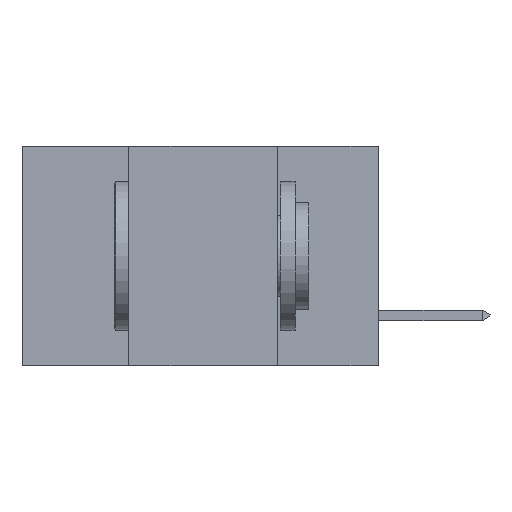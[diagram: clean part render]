
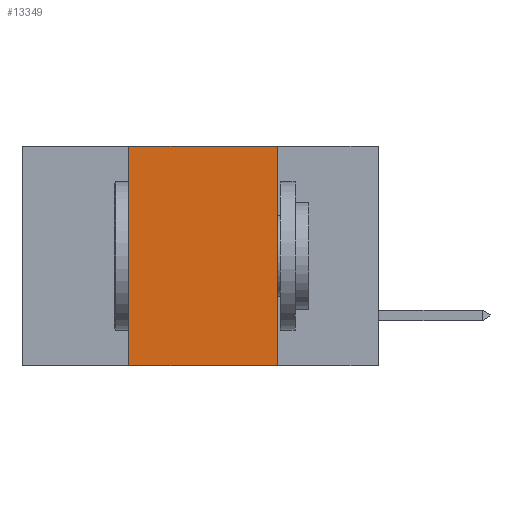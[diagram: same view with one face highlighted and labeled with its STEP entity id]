
A CAD part, left-side view. The second image highlights one B-rep face of the part: STEP entity #13349.
In plain terms, the highlighted planar face has unit normal (-1, 0, 0).
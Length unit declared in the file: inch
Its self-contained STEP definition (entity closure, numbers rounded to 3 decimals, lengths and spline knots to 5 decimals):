
#490 = DIRECTION ( 'NONE',  ( 0., 0., -1. ) ) ;
#607 = ORIENTED_EDGE ( 'NONE', *, *, #9971, .F. ) ;
#1518 = VECTOR ( 'NONE', #14403, 39.37008 ) ;
#1872 = CARTESIAN_POINT ( 'NONE',  ( 0., 0.17, -0.37 ) ) ;
#1937 = DIRECTION ( 'NONE',  ( 0., 0., 1. ) ) ;
#2011 = DIRECTION ( 'NONE',  ( 0., -1., 0. ) ) ;
#2223 = CARTESIAN_POINT ( 'NONE',  ( 0., 0.6, 0. ) ) ;
#2901 = CARTESIAN_POINT ( 'NONE',  ( 0., 0.6, -0.37 ) ) ;
#3441 = CARTESIAN_POINT ( 'NONE',  ( 0., 0.17, -0.37 ) ) ;
#4561 = EDGE_CURVE ( 'NONE', #14343, #15973, #16982, .T. ) ;
#4837 = CARTESIAN_POINT ( 'NONE',  ( 0., 0.6, 0. ) ) ;
#4923 = CARTESIAN_POINT ( 'NONE',  ( 0., 0.42, -0.37 ) ) ;
#4926 = PLANE ( 'NONE',  #6659 ) ;
#5362 = LINE ( 'NONE', #1872, #1518 ) ;
#6659 = AXIS2_PLACEMENT_3D ( 'NONE', #4837, #17475, #490 ) ;
#7638 = VECTOR ( 'NONE', #2011, 39.37008 ) ;
#7945 = VECTOR ( 'NONE', #1937, 39.37008 ) ;
#8205 = EDGE_CURVE ( 'NONE', #14343, #11895, #14176, .T. ) ;
#8904 = EDGE_LOOP ( 'NONE', ( #15608, #607, #11884, #18557 ) ) ;
#9418 = CARTESIAN_POINT ( 'NONE',  ( 0., 0.42, -0.37 ) ) ;
#9971 = EDGE_CURVE ( 'NONE', #11895, #12673, #14649, .T. ) ;
#10151 = VECTOR ( 'NONE', #17196, 39.37008 ) ;
#10498 = CARTESIAN_POINT ( 'NONE',  ( 0., 0.42, 0. ) ) ;
#11884 = ORIENTED_EDGE ( 'NONE', *, *, #8205, .F. ) ;
#11895 = VERTEX_POINT ( 'NONE', #10498 ) ;
#12673 = VERTEX_POINT ( 'NONE', #13299 ) ;
#13299 = CARTESIAN_POINT ( 'NONE',  ( 0., 0.17, 0. ) ) ;
#13349 = ADVANCED_FACE ( 'NONE', ( #18923 ), #4926, .F. ) ;
#14176 = LINE ( 'NONE', #4923, #7945 ) ;
#14343 = VERTEX_POINT ( 'NONE', #9418 ) ;
#14403 = DIRECTION ( 'NONE',  ( 0., 0., -1. ) ) ;
#14646 = EDGE_CURVE ( 'NONE', #12673, #15973, #5362, .T. ) ;
#14649 = LINE ( 'NONE', #2223, #7638 ) ;
#15608 = ORIENTED_EDGE ( 'NONE', *, *, #14646, .F. ) ;
#15973 = VERTEX_POINT ( 'NONE', #3441 ) ;
#16982 = LINE ( 'NONE', #2901, #10151 ) ;
#17196 = DIRECTION ( 'NONE',  ( 0., -1., 0. ) ) ;
#17475 = DIRECTION ( 'NONE',  ( 1., 0., 0. ) ) ;
#18557 = ORIENTED_EDGE ( 'NONE', *, *, #4561, .T. ) ;
#18923 = FACE_OUTER_BOUND ( 'NONE', #8904, .T. ) ;
